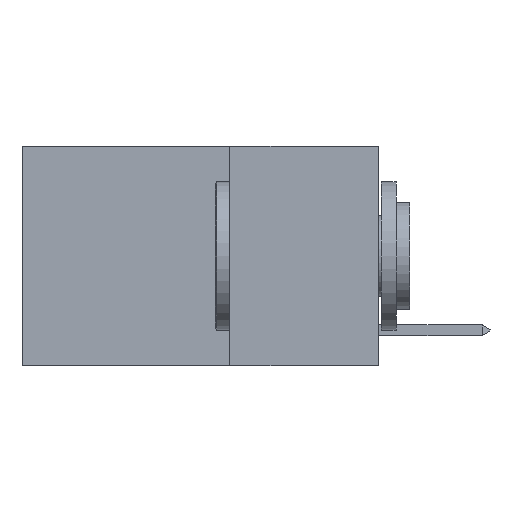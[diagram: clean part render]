
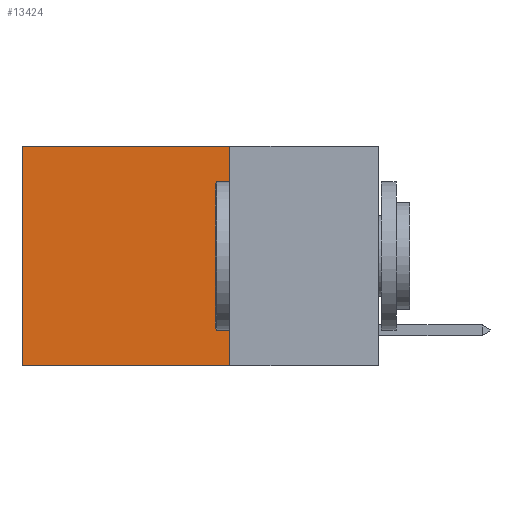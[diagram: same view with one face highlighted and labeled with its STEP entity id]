
A CAD part, left-side view. The second image highlights one B-rep face of the part: STEP entity #13424.
In plain terms, the highlighted planar face has unit normal (-1, 0, 0).
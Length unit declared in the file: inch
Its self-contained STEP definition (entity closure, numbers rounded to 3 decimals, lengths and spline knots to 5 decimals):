
#167 = EDGE_LOOP ( 'NONE', ( #9496, #20189, #1142, #3758 ) ) ;
#1051 = DIRECTION ( 'NONE',  ( 0., 1., 0. ) ) ;
#1142 = ORIENTED_EDGE ( 'NONE', *, *, #16072, .F. ) ;
#1440 = CARTESIAN_POINT ( 'NONE',  ( 0.2625, 0.25, 0. ) ) ;
#2851 = CARTESIAN_POINT ( 'NONE',  ( 0.2625, 0.25, -0.37 ) ) ;
#3015 = LINE ( 'NONE', #1440, #10834 ) ;
#3758 = ORIENTED_EDGE ( 'NONE', *, *, #7315, .T. ) ;
#6710 = AXIS2_PLACEMENT_3D ( 'NONE', #16826, #10591, #7230 ) ;
#7057 = CARTESIAN_POINT ( 'NONE',  ( 0.2625, 0.6, 0. ) ) ;
#7230 = DIRECTION ( 'NONE',  ( 0., 0., -1. ) ) ;
#7315 = EDGE_CURVE ( 'NONE', #19652, #9085, #10231, .T. ) ;
#7835 = DIRECTION ( 'NONE',  ( 0., 0., -1. ) ) ;
#8901 = PLANE ( 'NONE',  #6710 ) ;
#9085 = VERTEX_POINT ( 'NONE', #7057 ) ;
#9496 = ORIENTED_EDGE ( 'NONE', *, *, #10541, .T. ) ;
#10193 = VECTOR ( 'NONE', #7835, 39.37008 ) ;
#10231 = LINE ( 'NONE', #13305, #15541 ) ;
#10278 = CARTESIAN_POINT ( 'NONE',  ( 0.2625, 0.25, 0. ) ) ;
#10541 = EDGE_CURVE ( 'NONE', #9085, #20573, #17344, .T. ) ;
#10591 = DIRECTION ( 'NONE',  ( 1., 0., 0. ) ) ;
#10834 = VECTOR ( 'NONE', #16239, 39.37008 ) ;
#13004 = VECTOR ( 'NONE', #1051, 39.37008 ) ;
#13305 = CARTESIAN_POINT ( 'NONE',  ( 0.2625, 0.25, 0. ) ) ;
#13424 = ADVANCED_FACE ( 'NONE', ( #15238 ), #8901, .F. ) ;
#14985 = DIRECTION ( 'NONE',  ( 0., 1., 0. ) ) ;
#15238 = FACE_OUTER_BOUND ( 'NONE', #167, .T. ) ;
#15541 = VECTOR ( 'NONE', #14985, 39.37008 ) ;
#16072 = EDGE_CURVE ( 'NONE', #19652, #17577, #3015, .T. ) ;
#16239 = DIRECTION ( 'NONE',  ( 0., 0., -1. ) ) ;
#16826 = CARTESIAN_POINT ( 'NONE',  ( 0.2625, 0.25, 0. ) ) ;
#17344 = LINE ( 'NONE', #19366, #10193 ) ;
#17386 = CARTESIAN_POINT ( 'NONE',  ( 0.2625, 0.6, -0.37 ) ) ;
#17577 = VERTEX_POINT ( 'NONE', #20594 ) ;
#19366 = CARTESIAN_POINT ( 'NONE',  ( 0.2625, 0.6, 0. ) ) ;
#19652 = VERTEX_POINT ( 'NONE', #10278 ) ;
#19785 = EDGE_CURVE ( 'NONE', #17577, #20573, #20550, .T. ) ;
#20189 = ORIENTED_EDGE ( 'NONE', *, *, #19785, .F. ) ;
#20550 = LINE ( 'NONE', #2851, #13004 ) ;
#20573 = VERTEX_POINT ( 'NONE', #17386 ) ;
#20594 = CARTESIAN_POINT ( 'NONE',  ( 0.2625, 0.25, -0.37 ) ) ;
